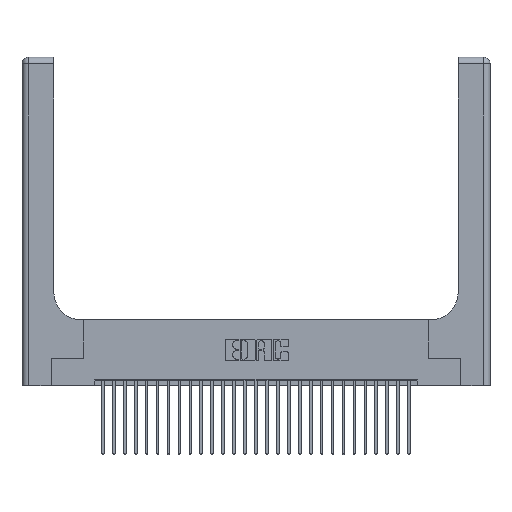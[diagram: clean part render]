
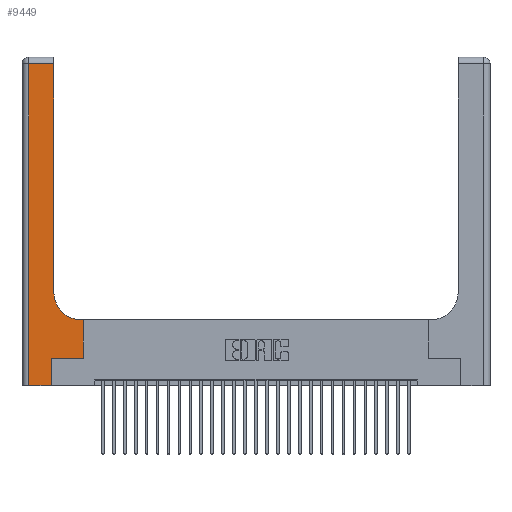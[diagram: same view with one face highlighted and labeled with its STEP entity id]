
A CAD part, top view. The second image highlights one B-rep face of the part: STEP entity #9449.
In plain terms, the highlighted planar face has unit normal (0, 0, 1).
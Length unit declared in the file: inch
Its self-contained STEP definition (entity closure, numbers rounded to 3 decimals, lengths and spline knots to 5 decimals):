
#1394 = FACE_OUTER_BOUND ( 'NONE', #16085, .T. ) ;
#1671 = CARTESIAN_POINT ( 'NONE',  ( 0.5585, 0.25, 0.37 ) ) ;
#1992 = DIRECTION ( 'NONE',  ( -1., 0., 0. ) ) ;
#2343 = VERTEX_POINT ( 'NONE', #24849 ) ;
#3812 = VECTOR ( 'NONE', #13514, 39.37008 ) ;
#3933 = VECTOR ( 'NONE', #11126, 39.37008 ) ;
#4004 = ORIENTED_EDGE ( 'NONE', *, *, #8718, .T. ) ;
#4166 = ORIENTED_EDGE ( 'NONE', *, *, #7077, .T. ) ;
#4403 = CARTESIAN_POINT ( 'NONE',  ( 0.5585, 0.25, 0.37 ) ) ;
#4602 = LINE ( 'NONE', #10877, #18901 ) ;
#4603 = EDGE_CURVE ( 'NONE', #10762, #6196, #29303, .T. ) ;
#6196 = VERTEX_POINT ( 'NONE', #9688 ) ;
#7077 = EDGE_CURVE ( 'NONE', #25401, #2343, #16872, .T. ) ;
#7407 = DIRECTION ( 'NONE',  ( 0., -1., 0. ) ) ;
#7508 = ORIENTED_EDGE ( 'NONE', *, *, #4603, .T. ) ;
#8143 = CARTESIAN_POINT ( 'NONE',  ( 0.2915, 0.6, 0.37 ) ) ;
#8389 = AXIS2_PLACEMENT_3D ( 'NONE', #12056, #25507, #14157 ) ;
#8718 = EDGE_CURVE ( 'NONE', #29682, #12019, #4602, .T. ) ;
#9417 = VECTOR ( 'NONE', #20713, 39.37008 ) ;
#9449 = ADVANCED_FACE ( 'NONE', ( #1394 ), #23209, .F. ) ;
#9688 = CARTESIAN_POINT ( 'NONE',  ( 0.5415, 0.6, 0.37 ) ) ;
#10762 = VERTEX_POINT ( 'NONE', #19054 ) ;
#10877 = CARTESIAN_POINT ( 'NONE',  ( 0., 2.94, 0.37 ) ) ;
#11067 = VERTEX_POINT ( 'NONE', #1671 ) ;
#11126 = DIRECTION ( 'NONE',  ( 1., 0., 0. ) ) ;
#12019 = VERTEX_POINT ( 'NONE', #19975 ) ;
#12056 = CARTESIAN_POINT ( 'NONE',  ( 0., 3., 0.37 ) ) ;
#12175 = CARTESIAN_POINT ( 'NONE',  ( 0.2915, 2.94, 0.37 ) ) ;
#12316 = VERTEX_POINT ( 'NONE', #14208 ) ;
#12631 = EDGE_CURVE ( 'NONE', #11067, #10762, #22357, .T. ) ;
#13292 = ORIENTED_EDGE ( 'NONE', *, *, #24315, .T. ) ;
#13514 = DIRECTION ( 'NONE',  ( 0., 1., 0. ) ) ;
#13844 = VECTOR ( 'NONE', #16533, 39.37008 ) ;
#13918 = CARTESIAN_POINT ( 'NONE',  ( 0.06, 3., 0.37 ) ) ;
#14157 = DIRECTION ( 'NONE',  ( -1., 0., 0. ) ) ;
#14179 = LINE ( 'NONE', #20235, #3812 ) ;
#14206 = CARTESIAN_POINT ( 'NONE',  ( 0.2915, 0.85, 0.37 ) ) ;
#14208 = CARTESIAN_POINT ( 'NONE',  ( 0.06, 0., 0.37 ) ) ;
#14390 = DIRECTION ( 'NONE',  ( 1., 0., 0. ) ) ;
#15977 = ORIENTED_EDGE ( 'NONE', *, *, #16495, .T. ) ;
#16085 = EDGE_LOOP ( 'NONE', ( #13292, #4004, #26474, #15977, #4166, #24359, #18047, #7508, #20953 ) ) ;
#16495 = EDGE_CURVE ( 'NONE', #12316, #25401, #16693, .T. ) ;
#16533 = DIRECTION ( 'NONE',  ( 1., 0., 0. ) ) ;
#16693 = LINE ( 'NONE', #25575, #13844 ) ;
#16872 = LINE ( 'NONE', #28265, #18635 ) ;
#17332 = DIRECTION ( 'NONE',  ( -1., 0., 0. ) ) ;
#18047 = ORIENTED_EDGE ( 'NONE', *, *, #12631, .T. ) ;
#18331 = CARTESIAN_POINT ( 'NONE',  ( 0.269, 0.25, 0.37 ) ) ;
#18635 = VECTOR ( 'NONE', #18863, 39.37008 ) ;
#18863 = DIRECTION ( 'NONE',  ( 0., 1., 0. ) ) ;
#18901 = VECTOR ( 'NONE', #1992, 39.37008 ) ;
#19054 = CARTESIAN_POINT ( 'NONE',  ( 0.5585, 0.6, 0.37 ) ) ;
#19975 = CARTESIAN_POINT ( 'NONE',  ( 0.06, 2.94, 0.37 ) ) ;
#20235 = CARTESIAN_POINT ( 'NONE',  ( 0.2915, 3., 0.37 ) ) ;
#20713 = DIRECTION ( 'NONE',  ( 0., 1., 0. ) ) ;
#20953 = ORIENTED_EDGE ( 'NONE', *, *, #27645, .T. ) ;
#22166 = CARTESIAN_POINT ( 'NONE',  ( 0.269, 0., 0.37 ) ) ;
#22302 = EDGE_CURVE ( 'NONE', #2343, #11067, #23636, .T. ) ;
#22357 = LINE ( 'NONE', #4403, #9417 ) ;
#23209 = PLANE ( 'NONE',  #8389 ) ;
#23530 = CARTESIAN_POINT ( 'NONE',  ( 0.5415, 0.85, 0.37 ) ) ;
#23636 = LINE ( 'NONE', #18331, #3933 ) ;
#24315 = EDGE_CURVE ( 'NONE', #24461, #29682, #14179, .T. ) ;
#24359 = ORIENTED_EDGE ( 'NONE', *, *, #22302, .T. ) ;
#24461 = VERTEX_POINT ( 'NONE', #14206 ) ;
#24849 = CARTESIAN_POINT ( 'NONE',  ( 0.269, 0.25, 0.37 ) ) ;
#25401 = VERTEX_POINT ( 'NONE', #22166 ) ;
#25507 = DIRECTION ( 'NONE',  ( 0., 0., -1. ) ) ;
#25575 = CARTESIAN_POINT ( 'NONE',  ( 0., 0., 0.37 ) ) ;
#25652 = VECTOR ( 'NONE', #17332, 39.37008 ) ;
#25837 = DIRECTION ( 'NONE',  ( 0., 0., -1. ) ) ;
#25925 = AXIS2_PLACEMENT_3D ( 'NONE', #23530, #25837, #14390 ) ;
#26474 = ORIENTED_EDGE ( 'NONE', *, *, #28959, .T. ) ;
#27231 = CIRCLE ( 'NONE', #25925, 0.25 ) ;
#27645 = EDGE_CURVE ( 'NONE', #6196, #24461, #27231, .T. ) ;
#28265 = CARTESIAN_POINT ( 'NONE',  ( 0.269, 0., 0.37 ) ) ;
#28959 = EDGE_CURVE ( 'NONE', #12019, #12316, #29338, .T. ) ;
#29303 = LINE ( 'NONE', #8143, #25652 ) ;
#29338 = LINE ( 'NONE', #13918, #29729 ) ;
#29682 = VERTEX_POINT ( 'NONE', #12175 ) ;
#29729 = VECTOR ( 'NONE', #7407, 39.37008 ) ;
